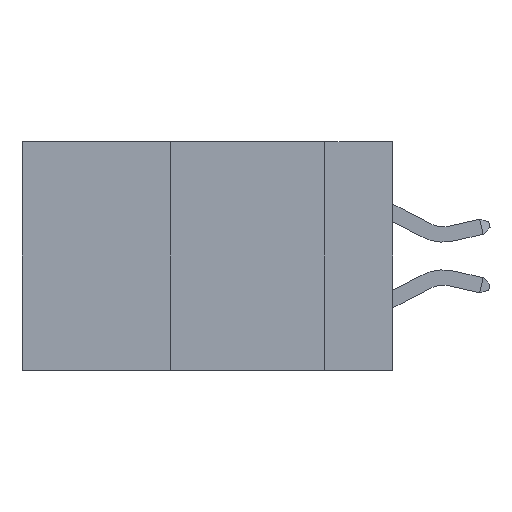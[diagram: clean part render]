
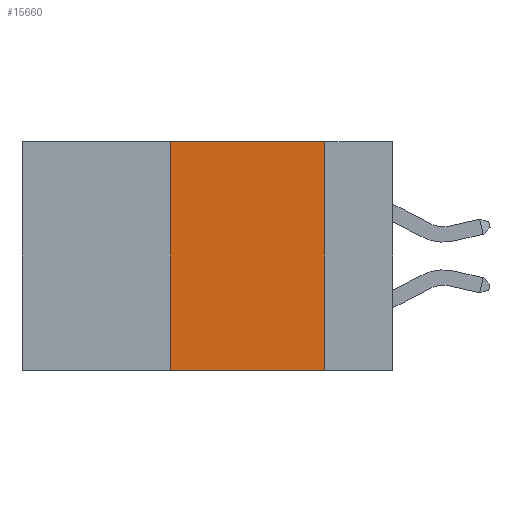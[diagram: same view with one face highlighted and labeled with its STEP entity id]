
A CAD part, left-side view. The second image highlights one B-rep face of the part: STEP entity #15660.
In plain terms, the highlighted planar face has unit normal (-1, 0, 0).
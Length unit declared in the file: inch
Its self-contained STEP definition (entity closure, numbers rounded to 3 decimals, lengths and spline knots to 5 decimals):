
#39 = ORIENTED_EDGE ( 'NONE', *, *, #8391, .T. ) ;
#74 = VECTOR ( 'NONE', #16845, 39.37008 ) ;
#668 = EDGE_CURVE ( 'NONE', #19073, #8049, #19362, .T. ) ;
#2087 = VERTEX_POINT ( 'NONE', #2661 ) ;
#2661 = CARTESIAN_POINT ( 'NONE',  ( 0., 0.36, 0. ) ) ;
#2840 = DIRECTION ( 'NONE',  ( 0., 0., 1. ) ) ;
#4440 = DIRECTION ( 'NONE',  ( 0., 0., -1. ) ) ;
#4450 = FACE_OUTER_BOUND ( 'NONE', #12585, .T. ) ;
#4762 = EDGE_CURVE ( 'NONE', #18909, #2087, #6312, .T. ) ;
#6312 = LINE ( 'NONE', #12253, #10022 ) ;
#6773 = CARTESIAN_POINT ( 'NONE',  ( 0., 0.6, -0.37 ) ) ;
#6882 = VECTOR ( 'NONE', #17797, 39.37008 ) ;
#7290 = VECTOR ( 'NONE', #16525, 39.37008 ) ;
#7485 = CARTESIAN_POINT ( 'NONE',  ( 0., 0.6, 0. ) ) ;
#7858 = EDGE_CURVE ( 'NONE', #2087, #19073, #12611, .T. ) ;
#8049 = VERTEX_POINT ( 'NONE', #18551 ) ;
#8391 = EDGE_CURVE ( 'NONE', #18909, #8049, #14301, .T. ) ;
#9415 = CARTESIAN_POINT ( 'NONE',  ( 0., 0.36, -0.37 ) ) ;
#10022 = VECTOR ( 'NONE', #2840, 39.37008 ) ;
#12253 = CARTESIAN_POINT ( 'NONE',  ( 0., 0.36, 0. ) ) ;
#12268 = PLANE ( 'NONE',  #18636 ) ;
#12585 = EDGE_LOOP ( 'NONE', ( #18192, #12983, #19561, #39 ) ) ;
#12611 = LINE ( 'NONE', #15283, #74 ) ;
#12983 = ORIENTED_EDGE ( 'NONE', *, *, #7858, .F. ) ;
#13063 = CARTESIAN_POINT ( 'NONE',  ( 0., 0.11, 0. ) ) ;
#13848 = DIRECTION ( 'NONE',  ( 1., 0., 0. ) ) ;
#14158 = CARTESIAN_POINT ( 'NONE',  ( 0., 0.11, 0. ) ) ;
#14301 = LINE ( 'NONE', #6773, #6882 ) ;
#15283 = CARTESIAN_POINT ( 'NONE',  ( 0., 0.6, 0. ) ) ;
#15660 = ADVANCED_FACE ( 'NONE', ( #4450 ), #12268, .F. ) ;
#16525 = DIRECTION ( 'NONE',  ( 0., 0., -1. ) ) ;
#16845 = DIRECTION ( 'NONE',  ( 0., -1., 0. ) ) ;
#17797 = DIRECTION ( 'NONE',  ( 0., -1., 0. ) ) ;
#18192 = ORIENTED_EDGE ( 'NONE', *, *, #668, .F. ) ;
#18551 = CARTESIAN_POINT ( 'NONE',  ( 0., 0.11, -0.37 ) ) ;
#18636 = AXIS2_PLACEMENT_3D ( 'NONE', #7485, #13848, #4440 ) ;
#18909 = VERTEX_POINT ( 'NONE', #9415 ) ;
#19073 = VERTEX_POINT ( 'NONE', #13063 ) ;
#19362 = LINE ( 'NONE', #14158, #7290 ) ;
#19561 = ORIENTED_EDGE ( 'NONE', *, *, #4762, .F. ) ;
